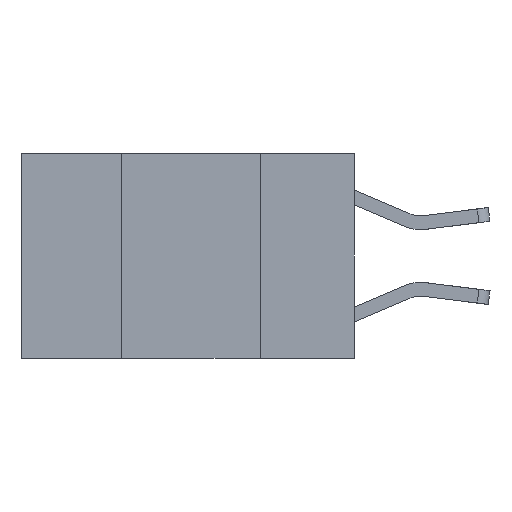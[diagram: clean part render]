
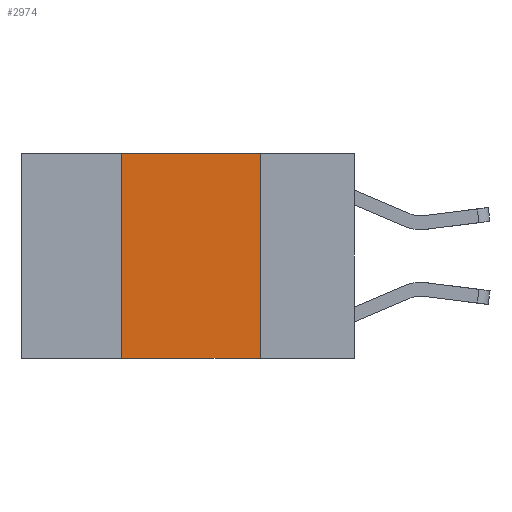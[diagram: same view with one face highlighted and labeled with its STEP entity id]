
A CAD part, left-side view. The second image highlights one B-rep face of the part: STEP entity #2974.
In plain terms, the highlighted planar face has unit normal (-1, 0, 0).
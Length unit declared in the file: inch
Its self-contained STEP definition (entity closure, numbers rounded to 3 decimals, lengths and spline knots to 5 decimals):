
#365 = DIRECTION ( 'NONE',  ( 0., 0., -1. ) ) ;
#436 = ORIENTED_EDGE ( 'NONE', *, *, #5029, .F. ) ;
#1041 = CARTESIAN_POINT ( 'NONE',  ( 0., 0.17, -0.37 ) ) ;
#1345 = CARTESIAN_POINT ( 'NONE',  ( 0., 0.17, 0. ) ) ;
#1404 = CARTESIAN_POINT ( 'NONE',  ( 0., 0.6, 0. ) ) ;
#1505 = DIRECTION ( 'NONE',  ( 0., -1., 0. ) ) ;
#1755 = DIRECTION ( 'NONE',  ( 0., 0., 1. ) ) ;
#2090 = LINE ( 'NONE', #11930, #6939 ) ;
#2165 = DIRECTION ( 'NONE',  ( 0., -1., 0. ) ) ;
#2195 = AXIS2_PLACEMENT_3D ( 'NONE', #1404, #8212, #2399 ) ;
#2399 = DIRECTION ( 'NONE',  ( 0., 0., -1. ) ) ;
#2725 = CARTESIAN_POINT ( 'NONE',  ( 0., 0.6, -0.37 ) ) ;
#2744 = VERTEX_POINT ( 'NONE', #1041 ) ;
#2974 = ADVANCED_FACE ( 'NONE', ( #3502 ), #12004, .F. ) ;
#3158 = VECTOR ( 'NONE', #1755, 39.37008 ) ;
#3502 = FACE_OUTER_BOUND ( 'NONE', #7055, .T. ) ;
#3589 = VERTEX_POINT ( 'NONE', #1345 ) ;
#4093 = EDGE_CURVE ( 'NONE', #10432, #3589, #12451, .T. ) ;
#5029 = EDGE_CURVE ( 'NONE', #3589, #2744, #2090, .T. ) ;
#5100 = EDGE_CURVE ( 'NONE', #7737, #2744, #8614, .T. ) ;
#5115 = EDGE_CURVE ( 'NONE', #7737, #10432, #5693, .T. ) ;
#5693 = LINE ( 'NONE', #6591, #3158 ) ;
#6322 = CARTESIAN_POINT ( 'NONE',  ( 0., 0.42, 0. ) ) ;
#6591 = CARTESIAN_POINT ( 'NONE',  ( 0., 0.42, 0. ) ) ;
#6939 = VECTOR ( 'NONE', #365, 39.37008 ) ;
#7055 = EDGE_LOOP ( 'NONE', ( #436, #11479, #7412, #12199 ) ) ;
#7398 = VECTOR ( 'NONE', #2165, 39.37008 ) ;
#7412 = ORIENTED_EDGE ( 'NONE', *, *, #5115, .F. ) ;
#7737 = VERTEX_POINT ( 'NONE', #7827 ) ;
#7827 = CARTESIAN_POINT ( 'NONE',  ( 0., 0.42, -0.37 ) ) ;
#7984 = CARTESIAN_POINT ( 'NONE',  ( 0., 0.6, 0. ) ) ;
#8212 = DIRECTION ( 'NONE',  ( 1., 0., 0. ) ) ;
#8614 = LINE ( 'NONE', #2725, #10884 ) ;
#10432 = VERTEX_POINT ( 'NONE', #6322 ) ;
#10884 = VECTOR ( 'NONE', #1505, 39.37008 ) ;
#11479 = ORIENTED_EDGE ( 'NONE', *, *, #4093, .F. ) ;
#11930 = CARTESIAN_POINT ( 'NONE',  ( 0., 0.17, 0. ) ) ;
#12004 = PLANE ( 'NONE',  #2195 ) ;
#12199 = ORIENTED_EDGE ( 'NONE', *, *, #5100, .T. ) ;
#12451 = LINE ( 'NONE', #7984, #7398 ) ;
